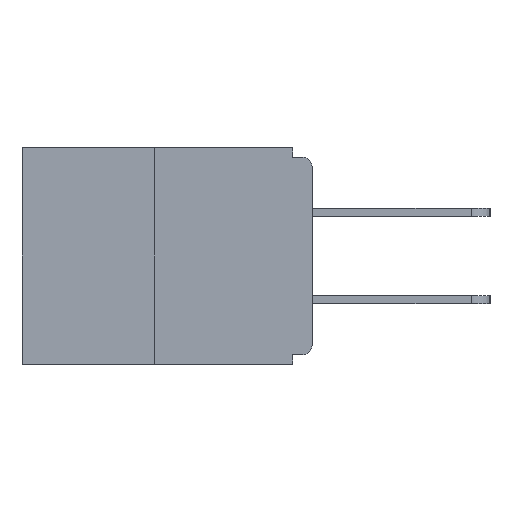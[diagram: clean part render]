
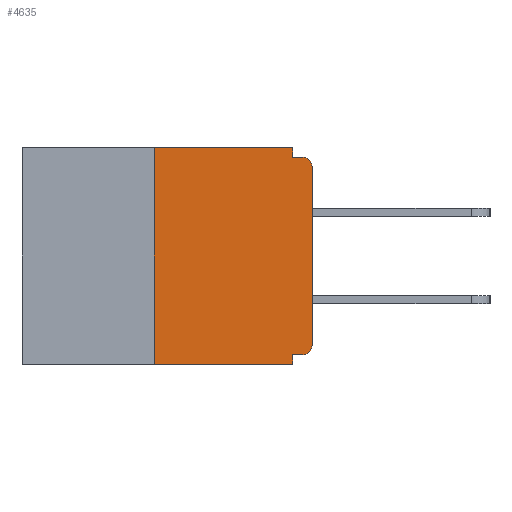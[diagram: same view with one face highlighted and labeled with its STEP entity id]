
A CAD part, left-side view. The second image highlights one B-rep face of the part: STEP entity #4635.
In plain terms, the highlighted planar face has unit normal (-1, 0, 0).
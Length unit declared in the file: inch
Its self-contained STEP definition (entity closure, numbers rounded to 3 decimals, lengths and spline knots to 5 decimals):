
#88 = ORIENTED_EDGE ( 'NONE', *, *, #17967, .T. ) ;
#307 = CARTESIAN_POINT ( 'NONE',  ( 0., 0.25, 0. ) ) ;
#485 = LINE ( 'NONE', #6751, #9295 ) ;
#721 = ORIENTED_EDGE ( 'NONE', *, *, #11372, .T. ) ;
#1567 = VECTOR ( 'NONE', #14508, 39.37008 ) ;
#1674 = EDGE_CURVE ( 'NONE', #4012, #16082, #18272, .T. ) ;
#1780 = EDGE_CURVE ( 'NONE', #16485, #19169, #17336, .T. ) ;
#1956 = VERTEX_POINT ( 'NONE', #17153 ) ;
#2028 = EDGE_CURVE ( 'NONE', #14931, #1956, #11619, .T. ) ;
#2555 = AXIS2_PLACEMENT_3D ( 'NONE', #8163, #18811, #12759 ) ;
#2625 = VECTOR ( 'NONE', #16846, 39.37008 ) ;
#2634 = ORIENTED_EDGE ( 'NONE', *, *, #3952, .F. ) ;
#2903 = CARTESIAN_POINT ( 'NONE',  ( 0., 0.031, -0.328 ) ) ;
#3245 = CARTESIAN_POINT ( 'NONE',  ( 0., 0., -0.313 ) ) ;
#3952 = EDGE_CURVE ( 'NONE', #14545, #15315, #13683, .T. ) ;
#4012 = VERTEX_POINT ( 'NONE', #2903 ) ;
#4026 = DIRECTION ( 'NONE',  ( 0., -1., 0. ) ) ;
#4080 = VECTOR ( 'NONE', #18348, 39.37008 ) ;
#4635 = ADVANCED_FACE ( 'NONE', ( #15968 ), #10242, .F. ) ;
#4954 = DIRECTION ( 'NONE',  ( -1., 0., 0. ) ) ;
#4996 = ORIENTED_EDGE ( 'NONE', *, *, #1780, .T. ) ;
#5056 = CARTESIAN_POINT ( 'NONE',  ( 0., 0.031, -0.015 ) ) ;
#5560 = VECTOR ( 'NONE', #4026, 39.37008 ) ;
#5605 = CARTESIAN_POINT ( 'NONE',  ( 0., 0.46, 0. ) ) ;
#6031 = LINE ( 'NONE', #14139, #5560 ) ;
#6033 = CARTESIAN_POINT ( 'NONE',  ( 0., 0.031, -0.343 ) ) ;
#6341 = CARTESIAN_POINT ( 'NONE',  ( 0., 0., -0.03 ) ) ;
#6700 = ORIENTED_EDGE ( 'NONE', *, *, #17544, .F. ) ;
#6751 = CARTESIAN_POINT ( 'NONE',  ( 0., 0., -0.328 ) ) ;
#6934 = LINE ( 'NONE', #19742, #2625 ) ;
#7248 = DIRECTION ( 'NONE',  ( 1., 0., 0. ) ) ;
#7666 = ORIENTED_EDGE ( 'NONE', *, *, #17846, .F. ) ;
#7672 = ORIENTED_EDGE ( 'NONE', *, *, #2028, .T. ) ;
#7822 = CARTESIAN_POINT ( 'NONE',  ( 0., 0.031, 0. ) ) ;
#8163 = CARTESIAN_POINT ( 'NONE',  ( 0., 0.015, -0.03 ) ) ;
#8343 = VECTOR ( 'NONE', #12528, 39.37008 ) ;
#8464 = DIRECTION ( 'NONE',  ( 0., 1., 0. ) ) ;
#8630 = ORIENTED_EDGE ( 'NONE', *, *, #11981, .F. ) ;
#8926 = CARTESIAN_POINT ( 'NONE',  ( 0., 0.25, 0. ) ) ;
#9295 = VECTOR ( 'NONE', #8464, 39.37008 ) ;
#10242 = PLANE ( 'NONE',  #15100 ) ;
#10458 = DIRECTION ( 'NONE',  ( 0., 0., 1. ) ) ;
#10518 = CARTESIAN_POINT ( 'NONE',  ( 0., 0.25, -0.343 ) ) ;
#10712 = LINE ( 'NONE', #13750, #4080 ) ;
#10777 = ORIENTED_EDGE ( 'NONE', *, *, #1674, .F. ) ;
#10982 = DIRECTION ( 'NONE',  ( 0., 0., -1. ) ) ;
#11134 = CARTESIAN_POINT ( 'NONE',  ( 0., 0., -0.015 ) ) ;
#11372 = EDGE_CURVE ( 'NONE', #18372, #16082, #6031, .T. ) ;
#11619 = CIRCLE ( 'NONE', #2555, 0.015 ) ;
#11861 = VECTOR ( 'NONE', #13569, 39.37008 ) ;
#11981 = EDGE_CURVE ( 'NONE', #16027, #1956, #14742, .T. ) ;
#12528 = DIRECTION ( 'NONE',  ( 0., -1., 0. ) ) ;
#12759 = DIRECTION ( 'NONE',  ( 0., 0., -1. ) ) ;
#13569 = DIRECTION ( 'NONE',  ( 0., 0., -1. ) ) ;
#13683 = LINE ( 'NONE', #19077, #1567 ) ;
#13750 = CARTESIAN_POINT ( 'NONE',  ( 0., 0., 0. ) ) ;
#13780 = VECTOR ( 'NONE', #10458, 39.37008 ) ;
#14139 = CARTESIAN_POINT ( 'NONE',  ( 0., 0.46, -0.343 ) ) ;
#14145 = CARTESIAN_POINT ( 'NONE',  ( 0., 0.015, -0.328 ) ) ;
#14235 = LINE ( 'NONE', #8926, #13780 ) ;
#14287 = EDGE_LOOP ( 'NONE', ( #2634, #7666, #721, #10777, #6700, #4996, #88, #7672, #8630, #18405 ) ) ;
#14431 = CARTESIAN_POINT ( 'NONE',  ( 0., 0.031, -0.343 ) ) ;
#14508 = DIRECTION ( 'NONE',  ( 0., -1., 0. ) ) ;
#14545 = VERTEX_POINT ( 'NONE', #307 ) ;
#14643 = DIRECTION ( 'NONE',  ( 0., 0., -1. ) ) ;
#14742 = LINE ( 'NONE', #11134, #8343 ) ;
#14931 = VERTEX_POINT ( 'NONE', #6341 ) ;
#15100 = AXIS2_PLACEMENT_3D ( 'NONE', #5605, #7248, #14643 ) ;
#15136 = CARTESIAN_POINT ( 'NONE',  ( 0., 0.015, -0.313 ) ) ;
#15315 = VERTEX_POINT ( 'NONE', #7822 ) ;
#15968 = FACE_OUTER_BOUND ( 'NONE', #14287, .T. ) ;
#16027 = VERTEX_POINT ( 'NONE', #5056 ) ;
#16082 = VERTEX_POINT ( 'NONE', #14431 ) ;
#16293 = EDGE_CURVE ( 'NONE', #15315, #16027, #6934, .T. ) ;
#16485 = VERTEX_POINT ( 'NONE', #14145 ) ;
#16846 = DIRECTION ( 'NONE',  ( 0., 0., -1. ) ) ;
#17153 = CARTESIAN_POINT ( 'NONE',  ( 0., 0.015, -0.015 ) ) ;
#17213 = AXIS2_PLACEMENT_3D ( 'NONE', #15136, #4954, #10982 ) ;
#17336 = CIRCLE ( 'NONE', #17213, 0.015 ) ;
#17544 = EDGE_CURVE ( 'NONE', #16485, #4012, #485, .T. ) ;
#17846 = EDGE_CURVE ( 'NONE', #18372, #14545, #14235, .T. ) ;
#17967 = EDGE_CURVE ( 'NONE', #19169, #14931, #10712, .T. ) ;
#18272 = LINE ( 'NONE', #6033, #11861 ) ;
#18348 = DIRECTION ( 'NONE',  ( 0., 0., 1. ) ) ;
#18372 = VERTEX_POINT ( 'NONE', #10518 ) ;
#18405 = ORIENTED_EDGE ( 'NONE', *, *, #16293, .F. ) ;
#18811 = DIRECTION ( 'NONE',  ( -1., 0., 0. ) ) ;
#19077 = CARTESIAN_POINT ( 'NONE',  ( 0., 0.46, 0. ) ) ;
#19169 = VERTEX_POINT ( 'NONE', #3245 ) ;
#19742 = CARTESIAN_POINT ( 'NONE',  ( 0., 0.031, 0. ) ) ;
